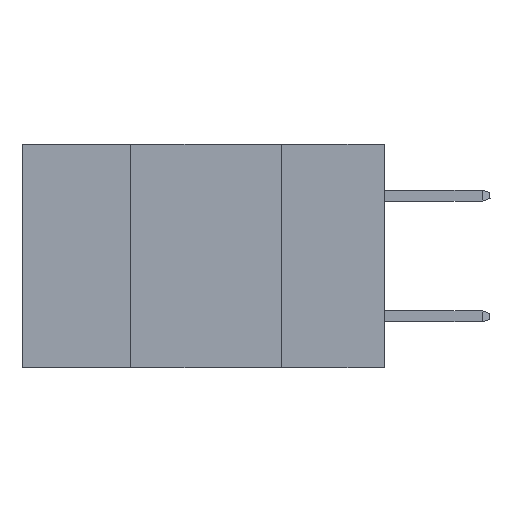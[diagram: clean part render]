
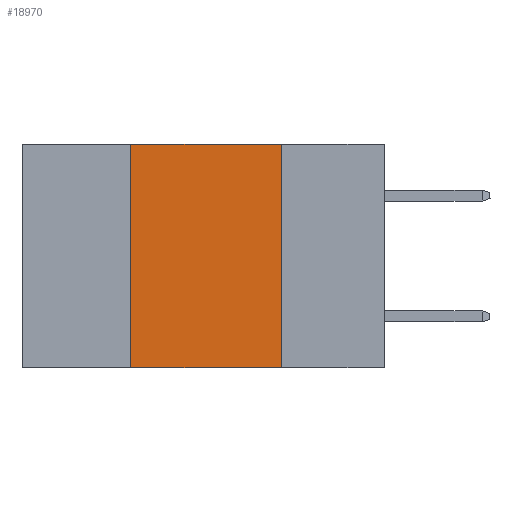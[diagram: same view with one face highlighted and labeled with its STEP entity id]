
A CAD part, left-side view. The second image highlights one B-rep face of the part: STEP entity #18970.
In plain terms, the highlighted planar face has unit normal (-1, 0, 0).
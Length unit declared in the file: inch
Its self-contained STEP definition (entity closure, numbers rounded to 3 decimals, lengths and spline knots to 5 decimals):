
#575 = CARTESIAN_POINT ( 'NONE',  ( 0., 0.6, -0.37 ) ) ;
#1245 = LINE ( 'NONE', #14338, #19629 ) ;
#1323 = ORIENTED_EDGE ( 'NONE', *, *, #13327, .F. ) ;
#1356 = VECTOR ( 'NONE', #5702, 39.37008 ) ;
#1611 = ORIENTED_EDGE ( 'NONE', *, *, #21204, .F. ) ;
#1656 = ORIENTED_EDGE ( 'NONE', *, *, #12172, .F. ) ;
#1797 = LINE ( 'NONE', #575, #10779 ) ;
#1811 = ORIENTED_EDGE ( 'NONE', *, *, #6164, .T. ) ;
#2548 = DIRECTION ( 'NONE',  ( 0., 0., 1. ) ) ;
#3402 = VECTOR ( 'NONE', #2548, 39.37008 ) ;
#3897 = AXIS2_PLACEMENT_3D ( 'NONE', #17724, #7066, #19478 ) ;
#5274 = PLANE ( 'NONE',  #3897 ) ;
#5537 = CARTESIAN_POINT ( 'NONE',  ( 0., 0.42, 0. ) ) ;
#5702 = DIRECTION ( 'NONE',  ( 0., 0., -1. ) ) ;
#6023 = VERTEX_POINT ( 'NONE', #5537 ) ;
#6164 = EDGE_CURVE ( 'NONE', #9380, #22158, #1797, .T. ) ;
#7066 = DIRECTION ( 'NONE',  ( 1., 0., 0. ) ) ;
#7867 = CARTESIAN_POINT ( 'NONE',  ( 0., 0.42, 0. ) ) ;
#9380 = VERTEX_POINT ( 'NONE', #13341 ) ;
#10779 = VECTOR ( 'NONE', #11327, 39.37008 ) ;
#10891 = LINE ( 'NONE', #16380, #1356 ) ;
#11327 = DIRECTION ( 'NONE',  ( 0., -1., 0. ) ) ;
#12172 = EDGE_CURVE ( 'NONE', #9380, #6023, #17610, .T. ) ;
#13327 = EDGE_CURVE ( 'NONE', #19029, #22158, #10891, .T. ) ;
#13341 = CARTESIAN_POINT ( 'NONE',  ( 0., 0.42, -0.37 ) ) ;
#14338 = CARTESIAN_POINT ( 'NONE',  ( 0., 0.6, 0. ) ) ;
#16043 = FACE_OUTER_BOUND ( 'NONE', #20461, .T. ) ;
#16130 = DIRECTION ( 'NONE',  ( 0., -1., 0. ) ) ;
#16380 = CARTESIAN_POINT ( 'NONE',  ( 0., 0.17, 0. ) ) ;
#17610 = LINE ( 'NONE', #7867, #3402 ) ;
#17724 = CARTESIAN_POINT ( 'NONE',  ( 0., 0.6, 0. ) ) ;
#17871 = CARTESIAN_POINT ( 'NONE',  ( 0., 0.17, 0. ) ) ;
#18970 = ADVANCED_FACE ( 'NONE', ( #16043 ), #5274, .F. ) ;
#19029 = VERTEX_POINT ( 'NONE', #17871 ) ;
#19478 = DIRECTION ( 'NONE',  ( 0., 0., -1. ) ) ;
#19629 = VECTOR ( 'NONE', #16130, 39.37008 ) ;
#20461 = EDGE_LOOP ( 'NONE', ( #1323, #1611, #1656, #1811 ) ) ;
#21204 = EDGE_CURVE ( 'NONE', #6023, #19029, #1245, .T. ) ;
#21989 = CARTESIAN_POINT ( 'NONE',  ( 0., 0.17, -0.37 ) ) ;
#22158 = VERTEX_POINT ( 'NONE', #21989 ) ;
